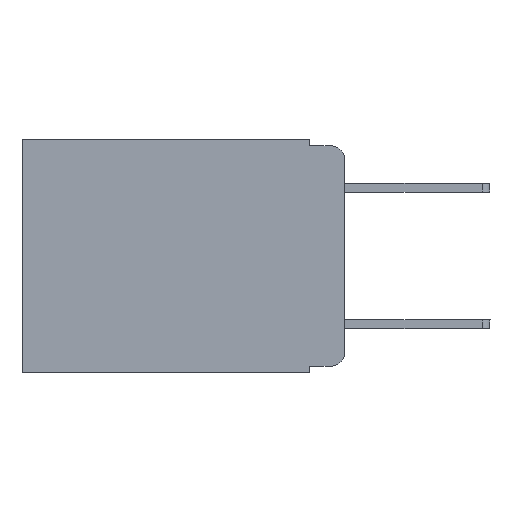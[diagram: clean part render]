
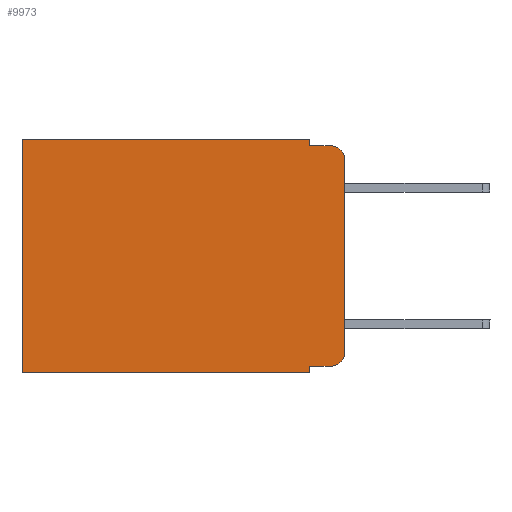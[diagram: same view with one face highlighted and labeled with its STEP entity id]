
A CAD part, left-side view. The second image highlights one B-rep face of the part: STEP entity #9973.
In plain terms, the highlighted planar face has unit normal (-1, 0, 0).
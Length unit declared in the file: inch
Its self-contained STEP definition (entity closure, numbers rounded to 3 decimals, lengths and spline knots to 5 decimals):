
#388 = CARTESIAN_POINT ( 'NONE',  ( 0.298, 0., 0. ) ) ;
#706 = DIRECTION ( 'NONE',  ( 0., -1., 0. ) ) ;
#809 = CARTESIAN_POINT ( 'NONE',  ( 0.298, 0., -0.343 ) ) ;
#865 = CARTESIAN_POINT ( 'NONE',  ( 0.298, 0.051, 0. ) ) ;
#1103 = VERTEX_POINT ( 'NONE', #10131 ) ;
#1341 = EDGE_LOOP ( 'NONE', ( #1517, #5073, #4603, #5417, #12511, #5868, #9594, #12779, #4362, #6710 ) ) ;
#1517 = ORIENTED_EDGE ( 'NONE', *, *, #6238, .F. ) ;
#1744 = AXIS2_PLACEMENT_3D ( 'NONE', #6265, #6160, #5153 ) ;
#2405 = VERTEX_POINT ( 'NONE', #3253 ) ;
#2863 = CARTESIAN_POINT ( 'NONE',  ( 0.298, 0.02, -0.01 ) ) ;
#2875 = EDGE_CURVE ( 'NONE', #2405, #7904, #10057, .T. ) ;
#3165 = LINE ( 'NONE', #388, #5998 ) ;
#3253 = CARTESIAN_POINT ( 'NONE',  ( 0.298, 0.473, 0. ) ) ;
#3628 = VERTEX_POINT ( 'NONE', #4920 ) ;
#3676 = CARTESIAN_POINT ( 'NONE',  ( 0.298, 0., -0.03 ) ) ;
#3720 = EDGE_CURVE ( 'NONE', #3628, #11298, #12524, .T. ) ;
#3906 = DIRECTION ( 'NONE',  ( 0., 0., -1. ) ) ;
#3946 = VECTOR ( 'NONE', #14310, 39.37008 ) ;
#3972 = CARTESIAN_POINT ( 'NONE',  ( 0.298, 0.051, -0.333 ) ) ;
#4215 = CARTESIAN_POINT ( 'NONE',  ( 0.298, 0.02, -0.313 ) ) ;
#4362 = ORIENTED_EDGE ( 'NONE', *, *, #10720, .T. ) ;
#4516 = CARTESIAN_POINT ( 'NONE',  ( 0.298, 0.473, -0.343 ) ) ;
#4603 = ORIENTED_EDGE ( 'NONE', *, *, #13507, .F. ) ;
#4817 = LINE ( 'NONE', #15471, #6496 ) ;
#4920 = CARTESIAN_POINT ( 'NONE',  ( 0.298, 0.02, -0.333 ) ) ;
#5020 = CARTESIAN_POINT ( 'NONE',  ( 0.298, 0.051, -0.01 ) ) ;
#5073 = ORIENTED_EDGE ( 'NONE', *, *, #9189, .T. ) ;
#5153 = DIRECTION ( 'NONE',  ( 0., 0., -1. ) ) ;
#5172 = DIRECTION ( 'NONE',  ( 0., -1., 0. ) ) ;
#5308 = VERTEX_POINT ( 'NONE', #2863 ) ;
#5417 = ORIENTED_EDGE ( 'NONE', *, *, #13540, .F. ) ;
#5517 = DIRECTION ( 'NONE',  ( 0., 0., -1. ) ) ;
#5707 = DIRECTION ( 'NONE',  ( 0., 1., 0. ) ) ;
#5868 = ORIENTED_EDGE ( 'NONE', *, *, #2875, .T. ) ;
#5998 = VECTOR ( 'NONE', #6339, 39.37008 ) ;
#6160 = DIRECTION ( 'NONE',  ( 1., 0., 0. ) ) ;
#6209 = LINE ( 'NONE', #9577, #3946 ) ;
#6238 = EDGE_CURVE ( 'NONE', #11757, #11298, #6209, .T. ) ;
#6265 = CARTESIAN_POINT ( 'NONE',  ( 0.298, 0., 0. ) ) ;
#6339 = DIRECTION ( 'NONE',  ( 0., 1., 0. ) ) ;
#6496 = VECTOR ( 'NONE', #13967, 39.37008 ) ;
#6710 = ORIENTED_EDGE ( 'NONE', *, *, #3720, .T. ) ;
#7185 = EDGE_CURVE ( 'NONE', #1103, #7904, #15038, .T. ) ;
#7293 = AXIS2_PLACEMENT_3D ( 'NONE', #11834, #11944, #12048 ) ;
#7417 = LINE ( 'NONE', #13845, #10990 ) ;
#7904 = VERTEX_POINT ( 'NONE', #4516 ) ;
#8044 = LINE ( 'NONE', #3972, #8621 ) ;
#8621 = VECTOR ( 'NONE', #5172, 39.37008 ) ;
#8626 = VECTOR ( 'NONE', #5707, 39.37008 ) ;
#8729 = CARTESIAN_POINT ( 'NONE',  ( 0.298, 0.473, 0. ) ) ;
#9189 = EDGE_CURVE ( 'NONE', #11757, #5308, #15105, .T. ) ;
#9577 = CARTESIAN_POINT ( 'NONE',  ( 0.298, 0., 0. ) ) ;
#9593 = FACE_OUTER_BOUND ( 'NONE', #1341, .T. ) ;
#9594 = ORIENTED_EDGE ( 'NONE', *, *, #7185, .F. ) ;
#9703 = LINE ( 'NONE', #13857, #13470 ) ;
#9973 = ADVANCED_FACE ( 'NONE', ( #9593 ), #14570, .F. ) ;
#10057 = LINE ( 'NONE', #8729, #14971 ) ;
#10131 = CARTESIAN_POINT ( 'NONE',  ( 0.298, 0.051, -0.343 ) ) ;
#10704 = EDGE_CURVE ( 'NONE', #12216, #2405, #3165, .T. ) ;
#10720 = EDGE_CURVE ( 'NONE', #10750, #3628, #8044, .T. ) ;
#10750 = VERTEX_POINT ( 'NONE', #14860 ) ;
#10990 = VECTOR ( 'NONE', #706, 39.37008 ) ;
#11091 = CARTESIAN_POINT ( 'NONE',  ( 0.298, 0., -0.313 ) ) ;
#11298 = VERTEX_POINT ( 'NONE', #11091 ) ;
#11757 = VERTEX_POINT ( 'NONE', #3676 ) ;
#11834 = CARTESIAN_POINT ( 'NONE',  ( 0.298, 0.02, -0.03 ) ) ;
#11944 = DIRECTION ( 'NONE',  ( -1., 0., 0. ) ) ;
#12048 = DIRECTION ( 'NONE',  ( 0., 0., -1. ) ) ;
#12216 = VERTEX_POINT ( 'NONE', #865 ) ;
#12480 = EDGE_CURVE ( 'NONE', #10750, #1103, #9703, .T. ) ;
#12511 = ORIENTED_EDGE ( 'NONE', *, *, #10704, .T. ) ;
#12524 = CIRCLE ( 'NONE', #15340, 0.02 ) ;
#12606 = VERTEX_POINT ( 'NONE', #5020 ) ;
#12779 = ORIENTED_EDGE ( 'NONE', *, *, #12480, .F. ) ;
#13470 = VECTOR ( 'NONE', #14927, 39.37008 ) ;
#13507 = EDGE_CURVE ( 'NONE', #12606, #5308, #7417, .T. ) ;
#13540 = EDGE_CURVE ( 'NONE', #12216, #12606, #4817, .T. ) ;
#13845 = CARTESIAN_POINT ( 'NONE',  ( 0.298, 0.051, -0.01 ) ) ;
#13857 = CARTESIAN_POINT ( 'NONE',  ( 0.298, 0.051, 0. ) ) ;
#13967 = DIRECTION ( 'NONE',  ( 0., 0., -1. ) ) ;
#14310 = DIRECTION ( 'NONE',  ( 0., 0., -1. ) ) ;
#14570 = PLANE ( 'NONE',  #1744 ) ;
#14860 = CARTESIAN_POINT ( 'NONE',  ( 0.298, 0.051, -0.333 ) ) ;
#14927 = DIRECTION ( 'NONE',  ( 0., 0., -1. ) ) ;
#14946 = DIRECTION ( 'NONE',  ( -1., 0., 0. ) ) ;
#14971 = VECTOR ( 'NONE', #3906, 39.37008 ) ;
#15038 = LINE ( 'NONE', #809, #8626 ) ;
#15105 = CIRCLE ( 'NONE', #7293, 0.02 ) ;
#15340 = AXIS2_PLACEMENT_3D ( 'NONE', #4215, #14946, #5517 ) ;
#15471 = CARTESIAN_POINT ( 'NONE',  ( 0.298, 0.051, 0. ) ) ;
